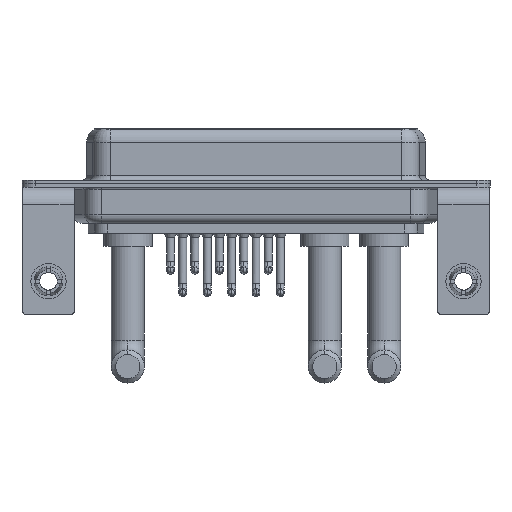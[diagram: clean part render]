
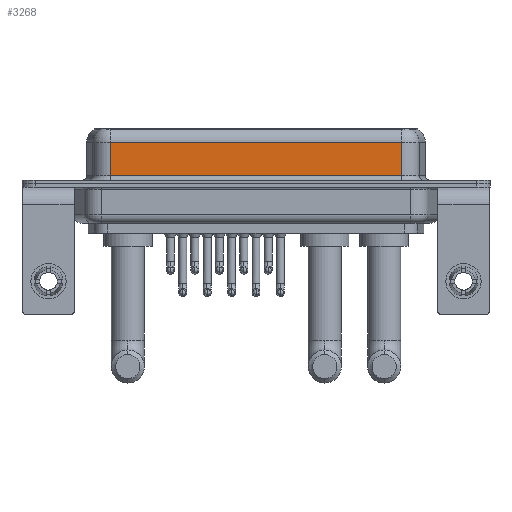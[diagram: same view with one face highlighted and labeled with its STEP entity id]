
A CAD part, front view. The second image highlights one B-rep face of the part: STEP entity #3268.
In plain terms, the highlighted planar face has unit normal (0, -1, 0).
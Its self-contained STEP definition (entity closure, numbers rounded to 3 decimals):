
#609 = ORIENTED_EDGE ( 'NONE', *, *, #11039, .F. ) ;
#867 = VECTOR ( 'NONE', #6312, 1000. ) ;
#892 = CARTESIAN_POINT ( 'NONE',  ( 7.013, -3.95, 6.4 ) ) ;
#1321 = CARTESIAN_POINT ( 'NONE',  ( 40.037, -3.95, 0.9 ) ) ;
#3268 = ADVANCED_FACE ( 'NONE', ( #16466 ), #13536, .F. ) ;
#3535 = CARTESIAN_POINT ( 'NONE',  ( 40.037, -3.95, 0.9 ) ) ;
#5344 = VERTEX_POINT ( 'NONE', #13919 ) ;
#6312 = DIRECTION ( 'NONE',  ( 1., 0., 0. ) ) ;
#7511 = DIRECTION ( 'NONE',  ( 0., 0., -1. ) ) ;
#8326 = DIRECTION ( 'NONE',  ( 0., 0., 1. ) ) ;
#8666 = CARTESIAN_POINT ( 'NONE',  ( 40.037, -3.95, 4.65 ) ) ;
#9581 = LINE ( 'NONE', #1321, #867 ) ;
#10936 = DIRECTION ( 'NONE',  ( 0., 0., -1. ) ) ;
#11039 = EDGE_CURVE ( 'NONE', #21428, #15323, #19186, .T. ) ;
#11489 = DIRECTION ( 'NONE',  ( 0., 1., 0. ) ) ;
#11641 = CARTESIAN_POINT ( 'NONE',  ( 40.037, -3.95, 4.65 ) ) ;
#12140 = CARTESIAN_POINT ( 'NONE',  ( 7.013, -3.95, 0.9 ) ) ;
#12858 = EDGE_CURVE ( 'NONE', #16659, #15323, #9581, .T. ) ;
#13226 = AXIS2_PLACEMENT_3D ( 'NONE', #13431, #11489, #8326 ) ;
#13431 = CARTESIAN_POINT ( 'NONE',  ( 40.037, -3.95, 6.4 ) ) ;
#13536 = PLANE ( 'NONE',  #13226 ) ;
#13919 = CARTESIAN_POINT ( 'NONE',  ( 7.013, -3.95, 4.65 ) ) ;
#14202 = CARTESIAN_POINT ( 'NONE',  ( 40.037, -3.95, 6.4 ) ) ;
#14570 = VECTOR ( 'NONE', #7511, 1000. ) ;
#15024 = VECTOR ( 'NONE', #10936, 1000. ) ;
#15294 = DIRECTION ( 'NONE',  ( -1., 0., 0. ) ) ;
#15323 = VERTEX_POINT ( 'NONE', #3535 ) ;
#15563 = VECTOR ( 'NONE', #15294, 1000. ) ;
#15718 = ORIENTED_EDGE ( 'NONE', *, *, #12858, .T. ) ;
#15767 = LINE ( 'NONE', #892, #14570 ) ;
#16466 = FACE_OUTER_BOUND ( 'NONE', #18747, .T. ) ;
#16659 = VERTEX_POINT ( 'NONE', #12140 ) ;
#17946 = EDGE_CURVE ( 'NONE', #21428, #5344, #19966, .T. ) ;
#18747 = EDGE_LOOP ( 'NONE', ( #609, #19259, #20279, #15718 ) ) ;
#19154 = EDGE_CURVE ( 'NONE', #5344, #16659, #15767, .T. ) ;
#19186 = LINE ( 'NONE', #14202, #15024 ) ;
#19259 = ORIENTED_EDGE ( 'NONE', *, *, #17946, .T. ) ;
#19966 = LINE ( 'NONE', #8666, #15563 ) ;
#20279 = ORIENTED_EDGE ( 'NONE', *, *, #19154, .T. ) ;
#21428 = VERTEX_POINT ( 'NONE', #11641 ) ;
